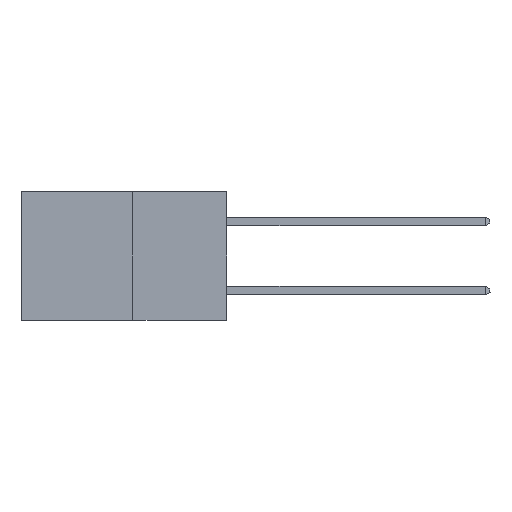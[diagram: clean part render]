
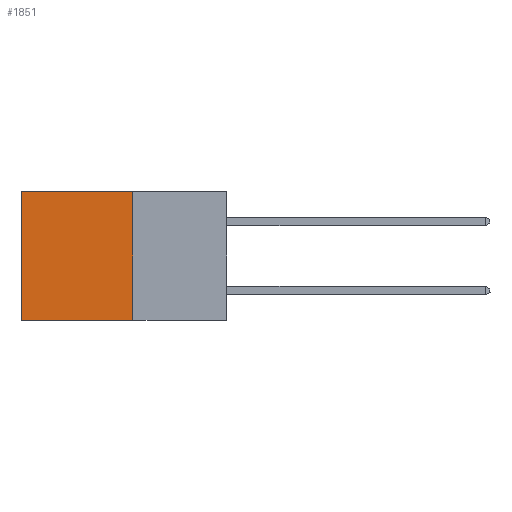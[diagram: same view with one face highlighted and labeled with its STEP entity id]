
A CAD part, left-side view. The second image highlights one B-rep face of the part: STEP entity #1851.
In plain terms, the highlighted planar face has unit normal (-1, 0, 0).
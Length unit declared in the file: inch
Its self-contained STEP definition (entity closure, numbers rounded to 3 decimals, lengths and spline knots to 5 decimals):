
#714 = CARTESIAN_POINT ( 'NONE',  ( 0.277, 0.59, -0.37 ) ) ;
#1851 = ADVANCED_FACE ( 'NONE', ( #4247 ), #7888, .F. ) ;
#2662 = LINE ( 'NONE', #18958, #10188 ) ;
#3153 = CARTESIAN_POINT ( 'NONE',  ( 0.277, 0.27, -0.37 ) ) ;
#3800 = DIRECTION ( 'NONE',  ( 0., 0., -1. ) ) ;
#3854 = CARTESIAN_POINT ( 'NONE',  ( 0.277, 0.59, 0. ) ) ;
#3871 = CARTESIAN_POINT ( 'NONE',  ( 0.277, 0.59, -0.37 ) ) ;
#4247 = FACE_OUTER_BOUND ( 'NONE', #15927, .T. ) ;
#5484 = DIRECTION ( 'NONE',  ( 0., 0., -1. ) ) ;
#5573 = ORIENTED_EDGE ( 'NONE', *, *, #13794, .F. ) ;
#6684 = DIRECTION ( 'NONE',  ( 1., 0., 0. ) ) ;
#6969 = VERTEX_POINT ( 'NONE', #3153 ) ;
#6983 = VECTOR ( 'NONE', #13982, 39.37008 ) ;
#7888 = PLANE ( 'NONE',  #15501 ) ;
#8266 = ORIENTED_EDGE ( 'NONE', *, *, #12478, .T. ) ;
#8435 = VECTOR ( 'NONE', #5484, 39.37008 ) ;
#8791 = CARTESIAN_POINT ( 'NONE',  ( 0.277, 0.27, -0.37 ) ) ;
#9083 = CARTESIAN_POINT ( 'NONE',  ( 0.277, 0.27, -0.37 ) ) ;
#10134 = LINE ( 'NONE', #8791, #17427 ) ;
#10188 = VECTOR ( 'NONE', #10289, 39.37008 ) ;
#10289 = DIRECTION ( 'NONE',  ( 0., 1., 0. ) ) ;
#10458 = VERTEX_POINT ( 'NONE', #3854 ) ;
#11153 = VERTEX_POINT ( 'NONE', #714 ) ;
#11211 = CARTESIAN_POINT ( 'NONE',  ( 0.277, 0.27, 0. ) ) ;
#11703 = VERTEX_POINT ( 'NONE', #11211 ) ;
#12476 = CARTESIAN_POINT ( 'NONE',  ( 0.277, 0.27, -0.37 ) ) ;
#12478 = EDGE_CURVE ( 'NONE', #11703, #10458, #2662, .T. ) ;
#13794 = EDGE_CURVE ( 'NONE', #11703, #6969, #10134, .T. ) ;
#13982 = DIRECTION ( 'NONE',  ( 0., 1., 0. ) ) ;
#14871 = EDGE_CURVE ( 'NONE', #6969, #11153, #18494, .T. ) ;
#15501 = AXIS2_PLACEMENT_3D ( 'NONE', #9083, #6684, #3800 ) ;
#15927 = EDGE_LOOP ( 'NONE', ( #15991, #17400, #5573, #8266 ) ) ;
#15991 = ORIENTED_EDGE ( 'NONE', *, *, #16272, .T. ) ;
#16014 = DIRECTION ( 'NONE',  ( 0., 0., -1. ) ) ;
#16272 = EDGE_CURVE ( 'NONE', #10458, #11153, #19000, .T. ) ;
#17400 = ORIENTED_EDGE ( 'NONE', *, *, #14871, .F. ) ;
#17427 = VECTOR ( 'NONE', #16014, 39.37008 ) ;
#18494 = LINE ( 'NONE', #12476, #6983 ) ;
#18958 = CARTESIAN_POINT ( 'NONE',  ( 0.277, 0.27, 0. ) ) ;
#19000 = LINE ( 'NONE', #3871, #8435 ) ;
